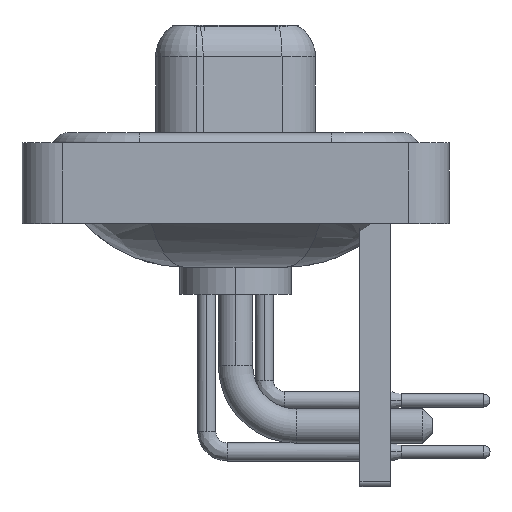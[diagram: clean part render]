
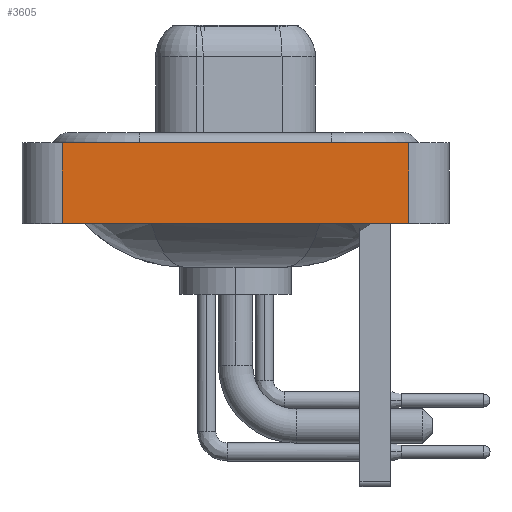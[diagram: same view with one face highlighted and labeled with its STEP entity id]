
A CAD part, left-side view. The second image highlights one B-rep face of the part: STEP entity #3605.
In plain terms, the highlighted planar face has unit normal (-1, 0, 0).
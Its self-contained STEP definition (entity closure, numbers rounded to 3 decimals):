
#334 = CARTESIAN_POINT ( 'NONE',  ( -7.35, -8.55, -3.6 ) ) ;
#438 = DIRECTION ( 'NONE',  ( -1., 0., 0. ) ) ;
#568 = VECTOR ( 'NONE', #21859, 1000. ) ;
#768 = ORIENTED_EDGE ( 'NONE', *, *, #16389, .F. ) ;
#1126 = DIRECTION ( 'NONE',  ( 0., 0., 1. ) ) ;
#1153 = ORIENTED_EDGE ( 'NONE', *, *, #17651, .F. ) ;
#1915 = VERTEX_POINT ( 'NONE', #14882 ) ;
#3560 = DIRECTION ( 'NONE',  ( 0., -1., 0. ) ) ;
#3605 = ADVANCED_FACE ( 'NONE', ( #21964 ), #4290, .T. ) ;
#4290 = PLANE ( 'NONE',  #15705 ) ;
#5658 = EDGE_LOOP ( 'NONE', ( #15401, #768, #1153, #23474 ) ) ;
#6477 = DIRECTION ( 'NONE',  ( 0., 0., 1. ) ) ;
#6508 = CARTESIAN_POINT ( 'NONE',  ( -7.35, -8.55, 0.4 ) ) ;
#6858 = LINE ( 'NONE', #24651, #13754 ) ;
#7149 = VECTOR ( 'NONE', #1126, 1000. ) ;
#7400 = EDGE_CURVE ( 'NONE', #11223, #1915, #6858, .T. ) ;
#8306 = LINE ( 'NONE', #334, #568 ) ;
#9688 = VERTEX_POINT ( 'NONE', #6508 ) ;
#9740 = CARTESIAN_POINT ( 'NONE',  ( -7.35, 8.55, -3.6 ) ) ;
#10902 = LINE ( 'NONE', #18769, #7149 ) ;
#11102 = DIRECTION ( 'NONE',  ( 0., -1., 0. ) ) ;
#11223 = VERTEX_POINT ( 'NONE', #9740 ) ;
#12139 = CARTESIAN_POINT ( 'NONE',  ( -7.35, -8.55, -3.6 ) ) ;
#12865 = CARTESIAN_POINT ( 'NONE',  ( -7.35, 8.55, 0.4 ) ) ;
#13754 = VECTOR ( 'NONE', #11102, 1000. ) ;
#14882 = CARTESIAN_POINT ( 'NONE',  ( -7.35, -8.55, -3.6 ) ) ;
#15401 = ORIENTED_EDGE ( 'NONE', *, *, #17828, .T. ) ;
#15705 = AXIS2_PLACEMENT_3D ( 'NONE', #12139, #438, #6477 ) ;
#16389 = EDGE_CURVE ( 'NONE', #23843, #9688, #23284, .T. ) ;
#17651 = EDGE_CURVE ( 'NONE', #11223, #23843, #10902, .T. ) ;
#17688 = VECTOR ( 'NONE', #3560, 1000. ) ;
#17828 = EDGE_CURVE ( 'NONE', #1915, #9688, #8306, .T. ) ;
#18769 = CARTESIAN_POINT ( 'NONE',  ( -7.35, 8.55, -3.6 ) ) ;
#21859 = DIRECTION ( 'NONE',  ( 0., 0., 1. ) ) ;
#21964 = FACE_OUTER_BOUND ( 'NONE', #5658, .T. ) ;
#23162 = CARTESIAN_POINT ( 'NONE',  ( -7.35, -8.55, 0.4 ) ) ;
#23284 = LINE ( 'NONE', #23162, #17688 ) ;
#23474 = ORIENTED_EDGE ( 'NONE', *, *, #7400, .T. ) ;
#23843 = VERTEX_POINT ( 'NONE', #12865 ) ;
#24651 = CARTESIAN_POINT ( 'NONE',  ( -7.35, -8.55, -3.6 ) ) ;
